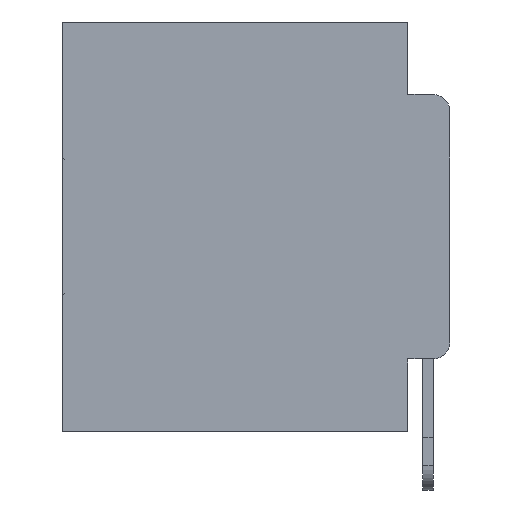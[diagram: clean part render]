
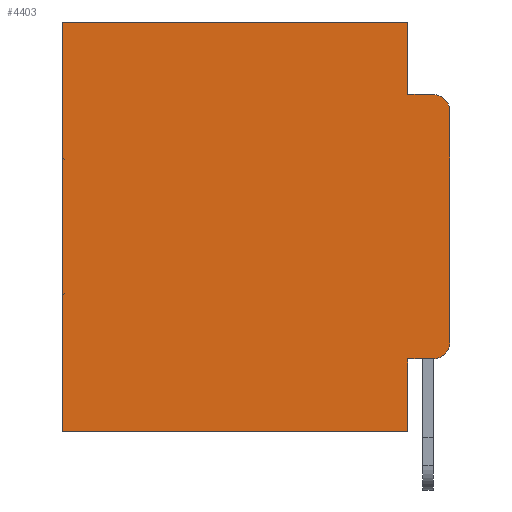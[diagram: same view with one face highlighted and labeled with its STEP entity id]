
A CAD part, left-side view. The second image highlights one B-rep face of the part: STEP entity #4403.
In plain terms, the highlighted planar face has unit normal (-1, 0, 0).
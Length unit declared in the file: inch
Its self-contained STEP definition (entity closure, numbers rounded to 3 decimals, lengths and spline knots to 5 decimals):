
#127 = VERTEX_POINT ( 'NONE', #7976 ) ;
#178 = LINE ( 'NONE', #11476, #25541 ) ;
#198 = CARTESIAN_POINT ( 'NONE',  ( 0.298, 0.473, 0. ) ) ;
#1281 = DIRECTION ( 'NONE',  ( 1., 0., 0. ) ) ;
#1447 = CARTESIAN_POINT ( 'NONE',  ( 0.298, 0.02, -0.3915 ) ) ;
#1472 = ORIENTED_EDGE ( 'NONE', *, *, #27199, .F. ) ;
#1817 = ORIENTED_EDGE ( 'NONE', *, *, #8393, .T. ) ;
#1863 = LINE ( 'NONE', #4441, #14609 ) ;
#1932 = EDGE_CURVE ( 'NONE', #7160, #7536, #13319, .T. ) ;
#2243 = CARTESIAN_POINT ( 'NONE',  ( 0.298, 0.051, -0.4115 ) ) ;
#2379 = CARTESIAN_POINT ( 'NONE',  ( 0.298, 0.051, 0. ) ) ;
#2411 = EDGE_CURVE ( 'NONE', #5733, #7160, #9386, .T. ) ;
#2623 = CARTESIAN_POINT ( 'NONE',  ( 0.298, 0., 0. ) ) ;
#2815 = PLANE ( 'NONE',  #24617 ) ;
#2910 = ORIENTED_EDGE ( 'NONE', *, *, #2411, .T. ) ;
#2982 = ORIENTED_EDGE ( 'NONE', *, *, #9179, .T. ) ;
#3038 = CARTESIAN_POINT ( 'NONE',  ( 0.298, 0.473, 0. ) ) ;
#3308 = VECTOR ( 'NONE', #11673, 39.37008 ) ;
#3514 = ORIENTED_EDGE ( 'NONE', *, *, #11064, .F. ) ;
#3552 = DIRECTION ( 'NONE',  ( 0., 0., -1. ) ) ;
#3910 = ORIENTED_EDGE ( 'NONE', *, *, #20840, .F. ) ;
#4131 = DIRECTION ( 'NONE',  ( 0., 0., -1. ) ) ;
#4403 = ADVANCED_FACE ( 'NONE', ( #8564 ), #2815, .F. ) ;
#4441 = CARTESIAN_POINT ( 'NONE',  ( 0.298, 0.051, 0. ) ) ;
#4738 = DIRECTION ( 'NONE',  ( -1., 0., 0. ) ) ;
#4745 = LINE ( 'NONE', #8487, #29375 ) ;
#4813 = DIRECTION ( 'NONE',  ( 0., -1., 0. ) ) ;
#4946 = CARTESIAN_POINT ( 'NONE',  ( 0.298, 0.051, 0. ) ) ;
#5081 = ORIENTED_EDGE ( 'NONE', *, *, #21207, .F. ) ;
#5733 = VERTEX_POINT ( 'NONE', #2379 ) ;
#7076 = DIRECTION ( 'NONE',  ( 0., 0., -1. ) ) ;
#7160 = VERTEX_POINT ( 'NONE', #3038 ) ;
#7536 = VERTEX_POINT ( 'NONE', #28515 ) ;
#7604 = CARTESIAN_POINT ( 'NONE',  ( 0.298, 0., 0. ) ) ;
#7976 = CARTESIAN_POINT ( 'NONE',  ( 0.298, 0., -0.1085 ) ) ;
#8393 = EDGE_CURVE ( 'NONE', #30163, #15007, #29862, .T. ) ;
#8487 = CARTESIAN_POINT ( 'NONE',  ( 0.298, 0., -0.5 ) ) ;
#8564 = FACE_OUTER_BOUND ( 'NONE', #15428, .T. ) ;
#9179 = EDGE_CURVE ( 'NONE', #127, #29397, #27643, .T. ) ;
#9386 = LINE ( 'NONE', #7604, #3308 ) ;
#10001 = DIRECTION ( 'NONE',  ( 0., 0., -1. ) ) ;
#11064 = EDGE_CURVE ( 'NONE', #14811, #29397, #178, .T. ) ;
#11476 = CARTESIAN_POINT ( 'NONE',  ( 0.298, 0.051, -0.0885 ) ) ;
#11673 = DIRECTION ( 'NONE',  ( 0., 1., 0. ) ) ;
#11747 = LINE ( 'NONE', #4946, #22067 ) ;
#12194 = CARTESIAN_POINT ( 'NONE',  ( 0.298, 0.02, -0.0885 ) ) ;
#13134 = ORIENTED_EDGE ( 'NONE', *, *, #1932, .T. ) ;
#13157 = CARTESIAN_POINT ( 'NONE',  ( 0.298, 0., -0.3915 ) ) ;
#13319 = LINE ( 'NONE', #198, #26395 ) ;
#14500 = DIRECTION ( 'NONE',  ( 0., 0., -1. ) ) ;
#14566 = ORIENTED_EDGE ( 'NONE', *, *, #22835, .T. ) ;
#14609 = VECTOR ( 'NONE', #7076, 39.37008 ) ;
#14811 = VERTEX_POINT ( 'NONE', #29917 ) ;
#15007 = VERTEX_POINT ( 'NONE', #16646 ) ;
#15428 = EDGE_LOOP ( 'NONE', ( #3910, #2982, #3514, #5081, #2910, #13134, #18694, #1472, #1817, #14566 ) ) ;
#15505 = CARTESIAN_POINT ( 'NONE',  ( 0.298, 0., 0. ) ) ;
#15884 = VERTEX_POINT ( 'NONE', #19900 ) ;
#16646 = CARTESIAN_POINT ( 'NONE',  ( 0.298, 0.02, -0.4115 ) ) ;
#18676 = VECTOR ( 'NONE', #19907, 39.37008 ) ;
#18694 = ORIENTED_EDGE ( 'NONE', *, *, #21821, .F. ) ;
#18914 = DIRECTION ( 'NONE',  ( -1., 0., 0. ) ) ;
#19428 = CARTESIAN_POINT ( 'NONE',  ( 0.298, 0.02, -0.1085 ) ) ;
#19900 = CARTESIAN_POINT ( 'NONE',  ( 0.298, 0.051, -0.5 ) ) ;
#19907 = DIRECTION ( 'NONE',  ( 0., 0., -1. ) ) ;
#20840 = EDGE_CURVE ( 'NONE', #127, #29669, #30146, .T. ) ;
#21207 = EDGE_CURVE ( 'NONE', #5733, #14811, #1863, .T. ) ;
#21770 = DIRECTION ( 'NONE',  ( 0., 0., -1. ) ) ;
#21821 = EDGE_CURVE ( 'NONE', #15884, #7536, #4745, .T. ) ;
#22067 = VECTOR ( 'NONE', #10001, 39.37008 ) ;
#22376 = AXIS2_PLACEMENT_3D ( 'NONE', #1447, #18914, #4131 ) ;
#22825 = DIRECTION ( 'NONE',  ( 0., 1., 0. ) ) ;
#22835 = EDGE_CURVE ( 'NONE', #15007, #29669, #23996, .T. ) ;
#23205 = AXIS2_PLACEMENT_3D ( 'NONE', #19428, #4738, #21770 ) ;
#23220 = DIRECTION ( 'NONE',  ( 0., -1., 0. ) ) ;
#23825 = VECTOR ( 'NONE', #4813, 39.37008 ) ;
#23996 = CIRCLE ( 'NONE', #22376, 0.02 ) ;
#24617 = AXIS2_PLACEMENT_3D ( 'NONE', #15505, #1281, #14500 ) ;
#25541 = VECTOR ( 'NONE', #23220, 39.37008 ) ;
#26395 = VECTOR ( 'NONE', #3552, 39.37008 ) ;
#27199 = EDGE_CURVE ( 'NONE', #30163, #15884, #11747, .T. ) ;
#27643 = CIRCLE ( 'NONE', #23205, 0.02 ) ;
#28338 = CARTESIAN_POINT ( 'NONE',  ( 0.298, 0.051, -0.4115 ) ) ;
#28515 = CARTESIAN_POINT ( 'NONE',  ( 0.298, 0.473, -0.5 ) ) ;
#29375 = VECTOR ( 'NONE', #22825, 39.37008 ) ;
#29397 = VERTEX_POINT ( 'NONE', #12194 ) ;
#29669 = VERTEX_POINT ( 'NONE', #13157 ) ;
#29862 = LINE ( 'NONE', #2243, #23825 ) ;
#29917 = CARTESIAN_POINT ( 'NONE',  ( 0.298, 0.051, -0.0885 ) ) ;
#30146 = LINE ( 'NONE', #2623, #18676 ) ;
#30163 = VERTEX_POINT ( 'NONE', #28338 ) ;
